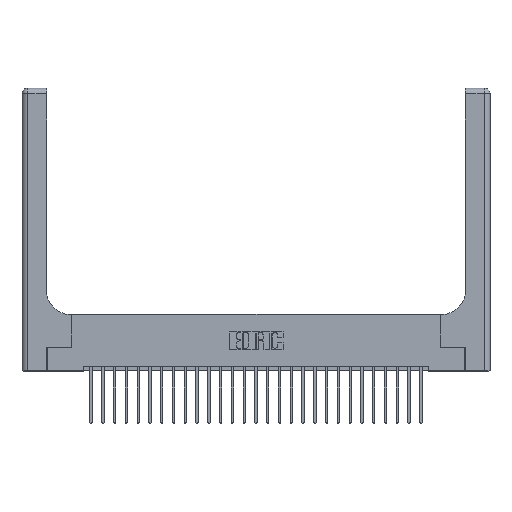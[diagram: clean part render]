
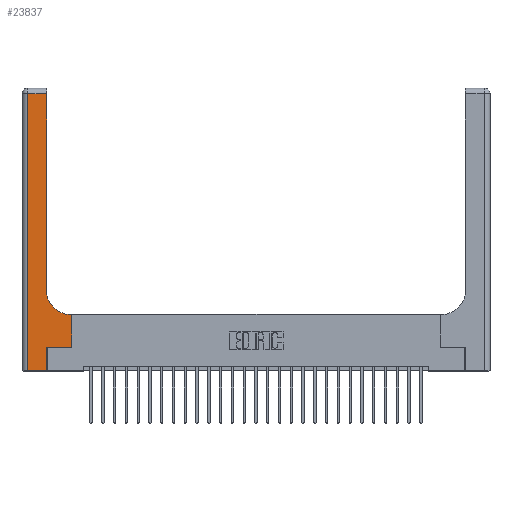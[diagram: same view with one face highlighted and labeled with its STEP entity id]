
A CAD part, top view. The second image highlights one B-rep face of the part: STEP entity #23837.
In plain terms, the highlighted planar face has unit normal (0, 0, 1).
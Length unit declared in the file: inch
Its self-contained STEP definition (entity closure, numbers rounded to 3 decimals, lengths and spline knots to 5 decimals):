
#89 = ORIENTED_EDGE ( 'NONE', *, *, #25744, .T. ) ;
#434 = VERTEX_POINT ( 'NONE', #12395 ) ;
#503 = DIRECTION ( 'NONE',  ( 1., 0., 0. ) ) ;
#1041 = EDGE_LOOP ( 'NONE', ( #20713, #14954, #3540, #11965, #6404, #5271, #3213, #5553, #89 ) ) ;
#1343 = DIRECTION ( 'NONE',  ( 1., 0., 0. ) ) ;
#1514 = LINE ( 'NONE', #10526, #12069 ) ;
#1749 = AXIS2_PLACEMENT_3D ( 'NONE', #23866, #11915, #2030 ) ;
#2030 = DIRECTION ( 'NONE',  ( 1., 0., 0. ) ) ;
#2033 = CARTESIAN_POINT ( 'NONE',  ( 0.06, 2.94, 0.37 ) ) ;
#2106 = CARTESIAN_POINT ( 'NONE',  ( 0., 3., 0.37 ) ) ;
#2183 = DIRECTION ( 'NONE',  ( 0., 0., -1. ) ) ;
#2436 = CARTESIAN_POINT ( 'NONE',  ( 0.26, 3., 0.37 ) ) ;
#3132 = VECTOR ( 'NONE', #503, 39.37008 ) ;
#3213 = ORIENTED_EDGE ( 'NONE', *, *, #11485, .T. ) ;
#3540 = ORIENTED_EDGE ( 'NONE', *, *, #4333, .T. ) ;
#3896 = VERTEX_POINT ( 'NONE', #15859 ) ;
#4068 = VECTOR ( 'NONE', #10144, 39.37008 ) ;
#4333 = EDGE_CURVE ( 'NONE', #17841, #3896, #9237, .T. ) ;
#5271 = ORIENTED_EDGE ( 'NONE', *, *, #11629, .T. ) ;
#5553 = ORIENTED_EDGE ( 'NONE', *, *, #16197, .T. ) ;
#5614 = LINE ( 'NONE', #8652, #3132 ) ;
#5798 = PLANE ( 'NONE',  #14038 ) ;
#5952 = CARTESIAN_POINT ( 'NONE',  ( 0.528, 0.25, 0.37 ) ) ;
#6312 = CARTESIAN_POINT ( 'NONE',  ( 0.26, 0.6, 0.37 ) ) ;
#6404 = ORIENTED_EDGE ( 'NONE', *, *, #21299, .T. ) ;
#7337 = CARTESIAN_POINT ( 'NONE',  ( 0.528, 0.6, 0.37 ) ) ;
#7400 = VERTEX_POINT ( 'NONE', #23593 ) ;
#8128 = VECTOR ( 'NONE', #8139, 39.37008 ) ;
#8139 = DIRECTION ( 'NONE',  ( 0., 1., 0. ) ) ;
#8478 = CARTESIAN_POINT ( 'NONE',  ( 0.265, 0., 0.37 ) ) ;
#8652 = CARTESIAN_POINT ( 'NONE',  ( 0.265, 0.25, 0.37 ) ) ;
#8932 = DIRECTION ( 'NONE',  ( 0., 1., 0. ) ) ;
#9237 = LINE ( 'NONE', #17656, #18579 ) ;
#10144 = DIRECTION ( 'NONE',  ( 0., 1., 0. ) ) ;
#10230 = CARTESIAN_POINT ( 'NONE',  ( 0.265, 0., 0.37 ) ) ;
#10474 = VERTEX_POINT ( 'NONE', #7337 ) ;
#10526 = CARTESIAN_POINT ( 'NONE',  ( 0., 2.94, 0.37 ) ) ;
#11485 = EDGE_CURVE ( 'NONE', #11931, #10474, #17154, .T. ) ;
#11574 = LINE ( 'NONE', #8478, #8128 ) ;
#11629 = EDGE_CURVE ( 'NONE', #24409, #11931, #5614, .T. ) ;
#11915 = DIRECTION ( 'NONE',  ( 0., 0., -1. ) ) ;
#11931 = VERTEX_POINT ( 'NONE', #19221 ) ;
#11965 = ORIENTED_EDGE ( 'NONE', *, *, #15732, .T. ) ;
#12069 = VECTOR ( 'NONE', #24495, 39.37008 ) ;
#12395 = CARTESIAN_POINT ( 'NONE',  ( 0.26, 0.85, 0.37 ) ) ;
#12579 = CARTESIAN_POINT ( 'NONE',  ( 0.26, 2.94, 0.37 ) ) ;
#12924 = VERTEX_POINT ( 'NONE', #10230 ) ;
#12996 = CIRCLE ( 'NONE', #1749, 0.25 ) ;
#13023 = LINE ( 'NONE', #6312, #23439 ) ;
#13945 = DIRECTION ( 'NONE',  ( 0., -1., 0. ) ) ;
#14038 = AXIS2_PLACEMENT_3D ( 'NONE', #2106, #2183, #17901 ) ;
#14954 = ORIENTED_EDGE ( 'NONE', *, *, #25165, .T. ) ;
#15732 = EDGE_CURVE ( 'NONE', #3896, #12924, #21867, .T. ) ;
#15859 = CARTESIAN_POINT ( 'NONE',  ( 0.06, 0., 0.37 ) ) ;
#16197 = EDGE_CURVE ( 'NONE', #10474, #7400, #13023, .T. ) ;
#16790 = CARTESIAN_POINT ( 'NONE',  ( 0., 0., 0.37 ) ) ;
#17154 = LINE ( 'NONE', #5952, #4068 ) ;
#17613 = CARTESIAN_POINT ( 'NONE',  ( 0.265, 0.25, 0.37 ) ) ;
#17656 = CARTESIAN_POINT ( 'NONE',  ( 0.06, 3., 0.37 ) ) ;
#17841 = VERTEX_POINT ( 'NONE', #2033 ) ;
#17901 = DIRECTION ( 'NONE',  ( -1., 0., 0. ) ) ;
#18018 = FACE_OUTER_BOUND ( 'NONE', #1041, .T. ) ;
#18579 = VECTOR ( 'NONE', #13945, 39.37008 ) ;
#19221 = CARTESIAN_POINT ( 'NONE',  ( 0.528, 0.25, 0.37 ) ) ;
#20713 = ORIENTED_EDGE ( 'NONE', *, *, #24014, .T. ) ;
#21299 = EDGE_CURVE ( 'NONE', #12924, #24409, #11574, .T. ) ;
#21483 = VERTEX_POINT ( 'NONE', #12579 ) ;
#21867 = LINE ( 'NONE', #16790, #24071 ) ;
#22126 = LINE ( 'NONE', #2436, #24677 ) ;
#23439 = VECTOR ( 'NONE', #24486, 39.37008 ) ;
#23593 = CARTESIAN_POINT ( 'NONE',  ( 0.51, 0.6, 0.37 ) ) ;
#23837 = ADVANCED_FACE ( 'NONE', ( #18018 ), #5798, .F. ) ;
#23866 = CARTESIAN_POINT ( 'NONE',  ( 0.51, 0.85, 0.37 ) ) ;
#24014 = EDGE_CURVE ( 'NONE', #434, #21483, #22126, .T. ) ;
#24071 = VECTOR ( 'NONE', #1343, 39.37008 ) ;
#24409 = VERTEX_POINT ( 'NONE', #17613 ) ;
#24486 = DIRECTION ( 'NONE',  ( -1., 0., 0. ) ) ;
#24495 = DIRECTION ( 'NONE',  ( -1., 0., 0. ) ) ;
#24677 = VECTOR ( 'NONE', #8932, 39.37008 ) ;
#25165 = EDGE_CURVE ( 'NONE', #21483, #17841, #1514, .T. ) ;
#25744 = EDGE_CURVE ( 'NONE', #7400, #434, #12996, .T. ) ;
